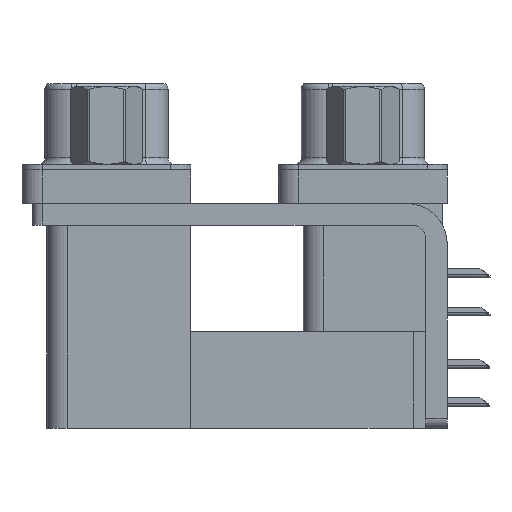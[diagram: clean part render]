
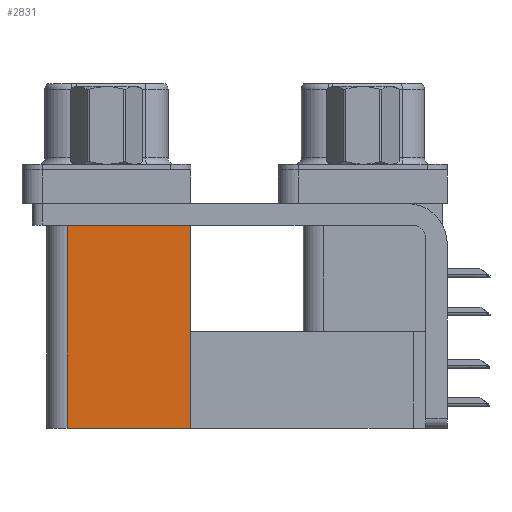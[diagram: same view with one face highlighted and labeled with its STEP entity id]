
A CAD part, left-side view. The second image highlights one B-rep face of the part: STEP entity #2831.
In plain terms, the highlighted planar face has unit normal (-1, 0, 0).
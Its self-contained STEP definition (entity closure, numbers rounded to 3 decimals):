
#303 = CARTESIAN_POINT ( 'NONE',  ( 3.765, 12.775, -19.2 ) ) ;
#1337 = LINE ( 'NONE', #29532, #35429 ) ;
#2131 = VERTEX_POINT ( 'NONE', #8594 ) ;
#2831 = ADVANCED_FACE ( 'NONE', ( #34000 ), #28143, .F. ) ;
#3032 = DIRECTION ( 'NONE',  ( 0., 0., -1. ) ) ;
#3866 = ORIENTED_EDGE ( 'NONE', *, *, #30881, .F. ) ;
#4799 = CARTESIAN_POINT ( 'NONE',  ( 3.765, 21.975, -2.5 ) ) ;
#5805 = DIRECTION ( 'NONE',  ( 0., 0., 1. ) ) ;
#7873 = AXIS2_PLACEMENT_3D ( 'NONE', #303, #26094, #3032 ) ;
#8525 = ORIENTED_EDGE ( 'NONE', *, *, #18661, .F. ) ;
#8594 = CARTESIAN_POINT ( 'NONE',  ( 3.765, 12.775, -19.2 ) ) ;
#9662 = EDGE_CURVE ( 'NONE', #2131, #24710, #10929, .T. ) ;
#10929 = LINE ( 'NONE', #22084, #30854 ) ;
#12504 = DIRECTION ( 'NONE',  ( 0., 1., 0. ) ) ;
#13693 = VECTOR ( 'NONE', #18486, 1000. ) ;
#14601 = CARTESIAN_POINT ( 'NONE',  ( 3.765, 21.975, -19.2 ) ) ;
#15334 = EDGE_LOOP ( 'NONE', ( #16543, #3866, #8525, #35042 ) ) ;
#16279 = LINE ( 'NONE', #24522, #13693 ) ;
#16543 = ORIENTED_EDGE ( 'NONE', *, *, #32726, .T. ) ;
#17316 = DIRECTION ( 'NONE',  ( 0., 0., 1. ) ) ;
#18486 = DIRECTION ( 'NONE',  ( 0., 1., 0. ) ) ;
#18661 = EDGE_CURVE ( 'NONE', #2131, #23322, #16279, .T. ) ;
#21593 = CARTESIAN_POINT ( 'NONE',  ( 3.765, 21.975, -19.2 ) ) ;
#22084 = CARTESIAN_POINT ( 'NONE',  ( 3.765, 12.775, -19.2 ) ) ;
#23322 = VERTEX_POINT ( 'NONE', #14601 ) ;
#24522 = CARTESIAN_POINT ( 'NONE',  ( 3.765, 12.775, -19.2 ) ) ;
#24710 = VERTEX_POINT ( 'NONE', #34460 ) ;
#25384 = VECTOR ( 'NONE', #5805, 1000. ) ;
#26094 = DIRECTION ( 'NONE',  ( 1., 0., 0. ) ) ;
#27511 = VERTEX_POINT ( 'NONE', #4799 ) ;
#28143 = PLANE ( 'NONE',  #7873 ) ;
#29532 = CARTESIAN_POINT ( 'NONE',  ( 3.765, 12.775, -2.5 ) ) ;
#30854 = VECTOR ( 'NONE', #17316, 1000. ) ;
#30881 = EDGE_CURVE ( 'NONE', #23322, #27511, #35501, .T. ) ;
#32726 = EDGE_CURVE ( 'NONE', #24710, #27511, #1337, .T. ) ;
#34000 = FACE_OUTER_BOUND ( 'NONE', #15334, .T. ) ;
#34460 = CARTESIAN_POINT ( 'NONE',  ( 3.765, 12.775, -2.5 ) ) ;
#35042 = ORIENTED_EDGE ( 'NONE', *, *, #9662, .T. ) ;
#35429 = VECTOR ( 'NONE', #12504, 1000. ) ;
#35501 = LINE ( 'NONE', #21593, #25384 ) ;
